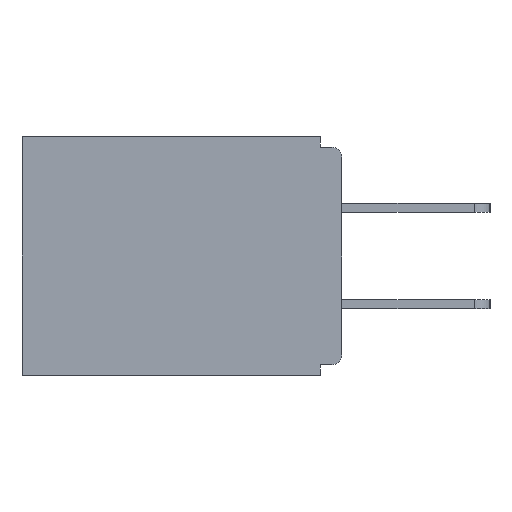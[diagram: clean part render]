
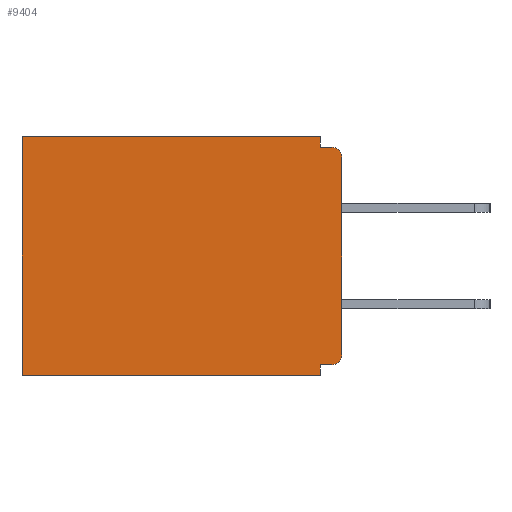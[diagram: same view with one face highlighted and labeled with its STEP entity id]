
A CAD part, left-side view. The second image highlights one B-rep face of the part: STEP entity #9404.
In plain terms, the highlighted planar face has unit normal (-1, 0, 0).
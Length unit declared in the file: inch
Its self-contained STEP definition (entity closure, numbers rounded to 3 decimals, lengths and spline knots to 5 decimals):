
#328 = ORIENTED_EDGE ( 'NONE', *, *, #7732, .F. ) ;
#489 = AXIS2_PLACEMENT_3D ( 'NONE', #17908, #8976, #16372 ) ;
#674 = DIRECTION ( 'NONE',  ( 0., 0., -1. ) ) ;
#837 = VECTOR ( 'NONE', #13995, 39.37008 ) ;
#958 = VECTOR ( 'NONE', #3756, 39.37008 ) ;
#986 = EDGE_CURVE ( 'NONE', #11661, #7206, #14241, .T. ) ;
#994 = VERTEX_POINT ( 'NONE', #10585 ) ;
#1553 = CARTESIAN_POINT ( 'NONE',  ( 0.298, 0., -0.328 ) ) ;
#1647 = LINE ( 'NONE', #17051, #12735 ) ;
#2569 = AXIS2_PLACEMENT_3D ( 'NONE', #9756, #5053, #674 ) ;
#2682 = VECTOR ( 'NONE', #2834, 39.37008 ) ;
#2759 = DIRECTION ( 'NONE',  ( 0., -1., 0. ) ) ;
#2834 = DIRECTION ( 'NONE',  ( 0., 1., 0. ) ) ;
#3724 = VECTOR ( 'NONE', #14091, 39.37008 ) ;
#3756 = DIRECTION ( 'NONE',  ( 0., 1., 0. ) ) ;
#4074 = ORIENTED_EDGE ( 'NONE', *, *, #986, .F. ) ;
#4370 = FACE_OUTER_BOUND ( 'NONE', #6903, .T. ) ;
#4512 = VERTEX_POINT ( 'NONE', #10050 ) ;
#5053 = DIRECTION ( 'NONE',  ( 1., 0., 0. ) ) ;
#6225 = VERTEX_POINT ( 'NONE', #15442 ) ;
#6339 = CARTESIAN_POINT ( 'NONE',  ( 0.298, 0.015, -0.328 ) ) ;
#6903 = EDGE_LOOP ( 'NONE', ( #12871, #8777, #7243, #8089, #9015, #328, #17943, #4074, #16913, #12003 ) ) ;
#6911 = CARTESIAN_POINT ( 'NONE',  ( 0.298, 0.015, -0.015 ) ) ;
#7206 = VERTEX_POINT ( 'NONE', #11501 ) ;
#7243 = ORIENTED_EDGE ( 'NONE', *, *, #16749, .F. ) ;
#7344 = VERTEX_POINT ( 'NONE', #9654 ) ;
#7732 = EDGE_CURVE ( 'NONE', #10803, #9749, #9262, .T. ) ;
#7739 = DIRECTION ( 'NONE',  ( 0., 0., -1. ) ) ;
#7861 = VECTOR ( 'NONE', #16037, 39.37008 ) ;
#8089 = ORIENTED_EDGE ( 'NONE', *, *, #18947, .T. ) ;
#8205 = CIRCLE ( 'NONE', #489, 0.015 ) ;
#8253 = EDGE_CURVE ( 'NONE', #994, #6225, #10177, .T. ) ;
#8294 = DIRECTION ( 'NONE',  ( -1., 0., 0. ) ) ;
#8406 = EDGE_CURVE ( 'NONE', #4512, #9749, #11101, .T. ) ;
#8777 = ORIENTED_EDGE ( 'NONE', *, *, #17538, .F. ) ;
#8976 = DIRECTION ( 'NONE',  ( -1., 0., 0. ) ) ;
#9015 = ORIENTED_EDGE ( 'NONE', *, *, #8406, .T. ) ;
#9262 = LINE ( 'NONE', #15847, #958 ) ;
#9404 = ADVANCED_FACE ( 'NONE', ( #4370 ), #11074, .F. ) ;
#9571 = VECTOR ( 'NONE', #7739, 39.37008 ) ;
#9654 = CARTESIAN_POINT ( 'NONE',  ( 0.298, 0.031, 0. ) ) ;
#9749 = VERTEX_POINT ( 'NONE', #10016 ) ;
#9756 = CARTESIAN_POINT ( 'NONE',  ( 0.298, 0., 0. ) ) ;
#9930 = VECTOR ( 'NONE', #10242, 39.37008 ) ;
#10016 = CARTESIAN_POINT ( 'NONE',  ( 0.298, 0.46, -0.343 ) ) ;
#10050 = CARTESIAN_POINT ( 'NONE',  ( 0.298, 0.46, 0. ) ) ;
#10177 = LINE ( 'NONE', #14655, #7861 ) ;
#10242 = DIRECTION ( 'NONE',  ( 0., 0., -1. ) ) ;
#10585 = CARTESIAN_POINT ( 'NONE',  ( 0.298, 0., -0.03 ) ) ;
#10803 = VERTEX_POINT ( 'NONE', #13183 ) ;
#10933 = EDGE_CURVE ( 'NONE', #11661, #6225, #8205, .T. ) ;
#11074 = PLANE ( 'NONE',  #2569 ) ;
#11101 = LINE ( 'NONE', #17817, #9930 ) ;
#11175 = EDGE_CURVE ( 'NONE', #994, #16375, #16071, .T. ) ;
#11253 = CARTESIAN_POINT ( 'NONE',  ( 0.298, 0., 0. ) ) ;
#11284 = DIRECTION ( 'NONE',  ( 0., 0., -1. ) ) ;
#11501 = CARTESIAN_POINT ( 'NONE',  ( 0.298, 0.031, -0.328 ) ) ;
#11661 = VERTEX_POINT ( 'NONE', #6339 ) ;
#12003 = ORIENTED_EDGE ( 'NONE', *, *, #8253, .F. ) ;
#12720 = LINE ( 'NONE', #11253, #3724 ) ;
#12735 = VECTOR ( 'NONE', #2759, 39.37008 ) ;
#12770 = CARTESIAN_POINT ( 'NONE',  ( 0.298, 0.031, -0.343 ) ) ;
#12871 = ORIENTED_EDGE ( 'NONE', *, *, #11175, .T. ) ;
#13034 = LINE ( 'NONE', #15058, #9571 ) ;
#13076 = LINE ( 'NONE', #12770, #837 ) ;
#13183 = CARTESIAN_POINT ( 'NONE',  ( 0.298, 0.031, -0.343 ) ) ;
#13587 = AXIS2_PLACEMENT_3D ( 'NONE', #14448, #8294, #11284 ) ;
#13995 = DIRECTION ( 'NONE',  ( 0., 0., -1. ) ) ;
#14091 = DIRECTION ( 'NONE',  ( 0., 1., 0. ) ) ;
#14241 = LINE ( 'NONE', #1553, #2682 ) ;
#14448 = CARTESIAN_POINT ( 'NONE',  ( 0.298, 0.015, -0.03 ) ) ;
#14655 = CARTESIAN_POINT ( 'NONE',  ( 0.298, 0., 0. ) ) ;
#15058 = CARTESIAN_POINT ( 'NONE',  ( 0.298, 0.031, -0.343 ) ) ;
#15442 = CARTESIAN_POINT ( 'NONE',  ( 0.298, 0., -0.313 ) ) ;
#15651 = VERTEX_POINT ( 'NONE', #18864 ) ;
#15847 = CARTESIAN_POINT ( 'NONE',  ( 0.298, 0., -0.343 ) ) ;
#16037 = DIRECTION ( 'NONE',  ( 0., 0., -1. ) ) ;
#16071 = CIRCLE ( 'NONE', #13587, 0.015 ) ;
#16372 = DIRECTION ( 'NONE',  ( 0., 0., -1. ) ) ;
#16375 = VERTEX_POINT ( 'NONE', #6911 ) ;
#16749 = EDGE_CURVE ( 'NONE', #7344, #15651, #13076, .T. ) ;
#16913 = ORIENTED_EDGE ( 'NONE', *, *, #10933, .T. ) ;
#17051 = CARTESIAN_POINT ( 'NONE',  ( 0.298, 0., -0.015 ) ) ;
#17228 = EDGE_CURVE ( 'NONE', #7206, #10803, #13034, .T. ) ;
#17538 = EDGE_CURVE ( 'NONE', #15651, #16375, #1647, .T. ) ;
#17817 = CARTESIAN_POINT ( 'NONE',  ( 0.298, 0.46, 0. ) ) ;
#17908 = CARTESIAN_POINT ( 'NONE',  ( 0.298, 0.015, -0.313 ) ) ;
#17943 = ORIENTED_EDGE ( 'NONE', *, *, #17228, .F. ) ;
#18864 = CARTESIAN_POINT ( 'NONE',  ( 0.298, 0.031, -0.015 ) ) ;
#18947 = EDGE_CURVE ( 'NONE', #7344, #4512, #12720, .T. ) ;
